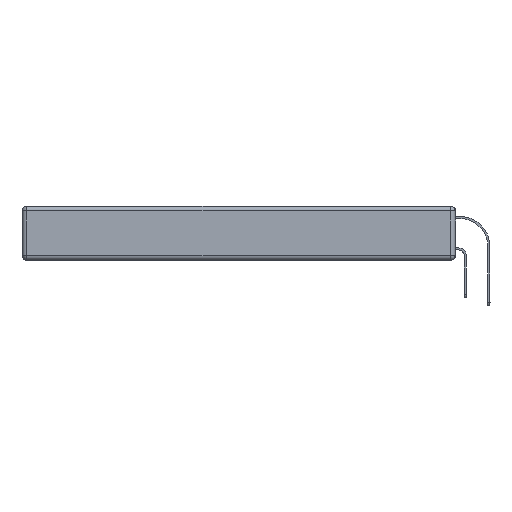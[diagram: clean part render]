
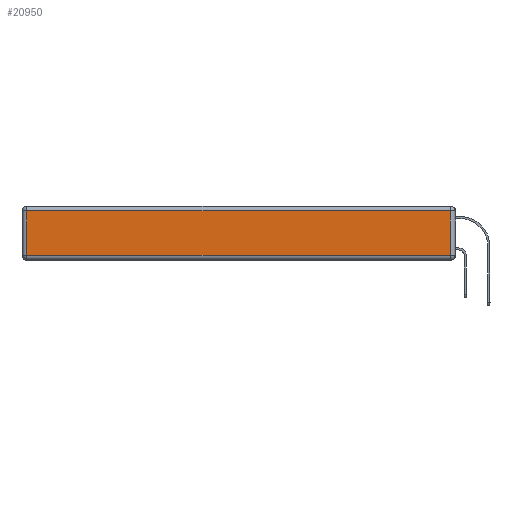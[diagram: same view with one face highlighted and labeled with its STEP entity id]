
A CAD part, left-side view. The second image highlights one B-rep face of the part: STEP entity #20950.
In plain terms, the highlighted planar face has unit normal (-1, 0, 0).
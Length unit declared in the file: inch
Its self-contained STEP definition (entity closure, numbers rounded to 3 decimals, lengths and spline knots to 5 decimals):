
#274 = EDGE_CURVE ( 'NONE', #8536, #9358, #6873, .T. ) ;
#906 = DIRECTION ( 'NONE',  ( -1., 0., 0. ) ) ;
#1053 = ORIENTED_EDGE ( 'NONE', *, *, #274, .T. ) ;
#1342 = EDGE_CURVE ( 'NONE', #6674, #22052, #3598, .T. ) ;
#1440 = DIRECTION ( 'NONE',  ( 0., 0., 1. ) ) ;
#2186 = VECTOR ( 'NONE', #15692, 39.37008 ) ;
#2592 = ORIENTED_EDGE ( 'NONE', *, *, #16301, .T. ) ;
#2770 = CARTESIAN_POINT ( 'NONE',  ( 0., 0., -0.343 ) ) ;
#2946 = ORIENTED_EDGE ( 'NONE', *, *, #1342, .T. ) ;
#3598 = LINE ( 'NONE', #11700, #2186 ) ;
#4572 = EDGE_CURVE ( 'NONE', #9358, #6674, #11173, .T. ) ;
#5277 = FACE_OUTER_BOUND ( 'NONE', #6575, .T. ) ;
#5461 = VECTOR ( 'NONE', #11382, 39.37008 ) ;
#5691 = LINE ( 'NONE', #21638, #13074 ) ;
#6575 = EDGE_LOOP ( 'NONE', ( #2946, #2592, #1053, #11913 ) ) ;
#6674 = VERTEX_POINT ( 'NONE', #17980 ) ;
#6873 = LINE ( 'NONE', #17491, #5461 ) ;
#7701 = CARTESIAN_POINT ( 'NONE',  ( 0., 0.03, -0.313 ) ) ;
#8536 = VERTEX_POINT ( 'NONE', #8887 ) ;
#8887 = CARTESIAN_POINT ( 'NONE',  ( 0., 0.03, -0.03 ) ) ;
#9358 = VERTEX_POINT ( 'NONE', #19042 ) ;
#11173 = LINE ( 'NONE', #17020, #15323 ) ;
#11382 = DIRECTION ( 'NONE',  ( 0., 1., 0. ) ) ;
#11518 = AXIS2_PLACEMENT_3D ( 'NONE', #2770, #906, #19233 ) ;
#11700 = CARTESIAN_POINT ( 'NONE',  ( 0., 0., -0.313 ) ) ;
#11913 = ORIENTED_EDGE ( 'NONE', *, *, #4572, .T. ) ;
#13074 = VECTOR ( 'NONE', #1440, 39.37008 ) ;
#13378 = PLANE ( 'NONE',  #11518 ) ;
#15279 = DIRECTION ( 'NONE',  ( 0., 0., -1. ) ) ;
#15323 = VECTOR ( 'NONE', #15279, 39.37008 ) ;
#15692 = DIRECTION ( 'NONE',  ( 0., -1., 0. ) ) ;
#16301 = EDGE_CURVE ( 'NONE', #22052, #8536, #5691, .T. ) ;
#17020 = CARTESIAN_POINT ( 'NONE',  ( 0., 2.72, -0.343 ) ) ;
#17491 = CARTESIAN_POINT ( 'NONE',  ( 0., 2.75, -0.03 ) ) ;
#17980 = CARTESIAN_POINT ( 'NONE',  ( 0., 2.72, -0.313 ) ) ;
#19042 = CARTESIAN_POINT ( 'NONE',  ( 0., 2.72, -0.03 ) ) ;
#19233 = DIRECTION ( 'NONE',  ( 0., 0., 1. ) ) ;
#20950 = ADVANCED_FACE ( 'NONE', ( #5277 ), #13378, .T. ) ;
#21638 = CARTESIAN_POINT ( 'NONE',  ( 0., 0.03, -0.343 ) ) ;
#22052 = VERTEX_POINT ( 'NONE', #7701 ) ;
